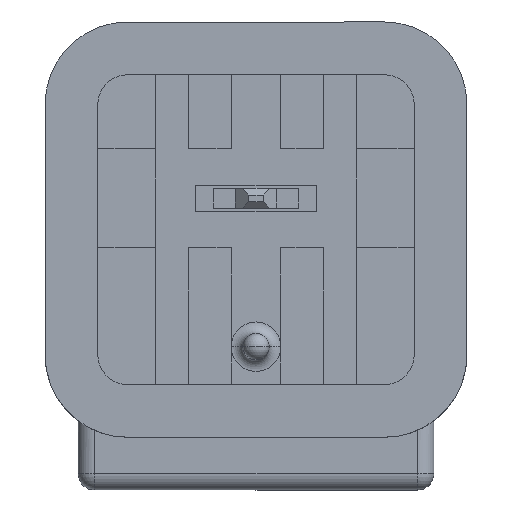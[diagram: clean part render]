
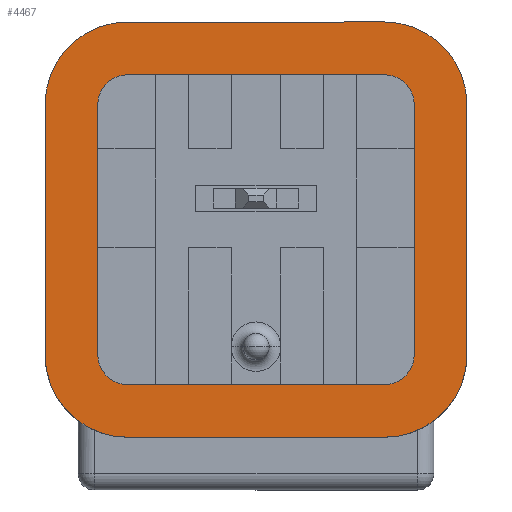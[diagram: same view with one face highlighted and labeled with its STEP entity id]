
A CAD part, front view. The second image highlights one B-rep face of the part: STEP entity #4467.
In plain terms, the highlighted planar face has unit normal (0, -1, 0).
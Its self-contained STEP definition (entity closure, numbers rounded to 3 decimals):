
#14 = LINE ( 'NONE', #4361, #474 ) ;
#16 = AXIS2_PLACEMENT_3D ( 'NONE', #4347, #647, #1285 ) ;
#30 = DIRECTION ( 'NONE',  ( 1., 0., 0. ) ) ;
#80 = EDGE_CURVE ( 'NONE', #1149, #186, #4325, .T. ) ;
#155 = DIRECTION ( 'NONE',  ( 0., -1., 0. ) ) ;
#169 = CIRCLE ( 'NONE', #16, 2.5 ) ;
#186 = VERTEX_POINT ( 'NONE', #326 ) ;
#187 = DIRECTION ( 'NONE',  ( 0., -1., 0. ) ) ;
#201 = EDGE_CURVE ( 'NONE', #4048, #1997, #14, .T. ) ;
#203 = ORIENTED_EDGE ( 'NONE', *, *, #2578, .F. ) ;
#245 = EDGE_LOOP ( 'NONE', ( #2085, #2388, #3092, #3180, #2538, #203, #2863, #3903 ) ) ;
#286 = CARTESIAN_POINT ( 'NONE',  ( -3.9, 0., -10.1 ) ) ;
#326 = CARTESIAN_POINT ( 'NONE',  ( 4.8, 0., -10.1 ) ) ;
#366 = CARTESIAN_POINT ( 'NONE',  ( 3.9, 0., -1.6 ) ) ;
#381 = CIRCLE ( 'NONE', #2443, 0.9 ) ;
#398 = VERTEX_POINT ( 'NONE', #4188 ) ;
#442 = VECTOR ( 'NONE', #2533, 1000. ) ;
#455 = EDGE_CURVE ( 'NONE', #3183, #1188, #4407, .T. ) ;
#460 = EDGE_CURVE ( 'NONE', #2556, #1149, #1193, .T. ) ;
#474 = VECTOR ( 'NONE', #3234, 1000. ) ;
#511 = VERTEX_POINT ( 'NONE', #2520 ) ;
#518 = ORIENTED_EDGE ( 'NONE', *, *, #4164, .F. ) ;
#536 = EDGE_CURVE ( 'NONE', #1997, #2963, #169, .T. ) ;
#548 = EDGE_CURVE ( 'NONE', #3319, #3502, #2851, .T. ) ;
#550 = AXIS2_PLACEMENT_3D ( 'NONE', #1909, #1558, #3824 ) ;
#595 = CARTESIAN_POINT ( 'NONE',  ( -3.9, 0., 0. ) ) ;
#647 = DIRECTION ( 'NONE',  ( 0., 1., 0. ) ) ;
#655 = EDGE_CURVE ( 'NONE', #1188, #3223, #761, .T. ) ;
#664 = CARTESIAN_POINT ( 'NONE',  ( -3.9, 0., -2.5 ) ) ;
#685 = EDGE_CURVE ( 'NONE', #2597, #398, #2942, .T. ) ;
#751 = ORIENTED_EDGE ( 'NONE', *, *, #3292, .F. ) ;
#761 = LINE ( 'NONE', #366, #1390 ) ;
#763 = CARTESIAN_POINT ( 'NONE',  ( 3.9, 0., -10.1 ) ) ;
#854 = DIRECTION ( 'NONE',  ( 1., 0., 0. ) ) ;
#877 = CARTESIAN_POINT ( 'NONE',  ( 3.9, 0., -1.6 ) ) ;
#903 = DIRECTION ( 'NONE',  ( 0., 1., 0. ) ) ;
#922 = EDGE_CURVE ( 'NONE', #3730, #4048, #2469, .T. ) ;
#946 = VERTEX_POINT ( 'NONE', #1386 ) ;
#964 = PLANE ( 'NONE',  #2120 ) ;
#981 = CARTESIAN_POINT ( 'NONE',  ( -3.9, 0., -12.6 ) ) ;
#999 = CIRCLE ( 'NONE', #2612, 2.5 ) ;
#1025 = CARTESIAN_POINT ( 'NONE',  ( -3.9, 0., -11. ) ) ;
#1032 = DIRECTION ( 'NONE',  ( -1., 0., 0. ) ) ;
#1072 = CARTESIAN_POINT ( 'NONE',  ( 6.4, 0., -10.1 ) ) ;
#1113 = VECTOR ( 'NONE', #4657, 1000. ) ;
#1137 = CARTESIAN_POINT ( 'NONE',  ( 6.4, 0., -2.5 ) ) ;
#1149 = VERTEX_POINT ( 'NONE', #1151 ) ;
#1151 = CARTESIAN_POINT ( 'NONE',  ( 3.9, 0., -11. ) ) ;
#1188 = VERTEX_POINT ( 'NONE', #877 ) ;
#1193 = LINE ( 'NONE', #4140, #3629 ) ;
#1254 = ORIENTED_EDGE ( 'NONE', *, *, #548, .F. ) ;
#1285 = DIRECTION ( 'NONE',  ( 1., 0., 0. ) ) ;
#1311 = DIRECTION ( 'NONE',  ( -1., 0., 0. ) ) ;
#1313 = CARTESIAN_POINT ( 'NONE',  ( -6.4, 0., -10.1 ) ) ;
#1386 = CARTESIAN_POINT ( 'NONE',  ( 6.4, 0., -10.1 ) ) ;
#1390 = VECTOR ( 'NONE', #2159, 1000. ) ;
#1432 = ORIENTED_EDGE ( 'NONE', *, *, #922, .F. ) ;
#1470 = CIRCLE ( 'NONE', #4695, 0.9 ) ;
#1491 = LINE ( 'NONE', #4414, #3271 ) ;
#1503 = CARTESIAN_POINT ( 'NONE',  ( -3.9, 0., 0. ) ) ;
#1558 = DIRECTION ( 'NONE',  ( 0., -1., 0. ) ) ;
#1606 = LINE ( 'NONE', #595, #1962 ) ;
#1729 = CARTESIAN_POINT ( 'NONE',  ( -3.9, 0., -1.6 ) ) ;
#1766 = DIRECTION ( 'NONE',  ( -1., 0., 0. ) ) ;
#1781 = DIRECTION ( 'NONE',  ( 1., 0., 0. ) ) ;
#1788 = ORIENTED_EDGE ( 'NONE', *, *, #2495, .F. ) ;
#1827 = CARTESIAN_POINT ( 'NONE',  ( 3.9, 0., -10.1 ) ) ;
#1868 = DIRECTION ( 'NONE',  ( 0., 0., 1. ) ) ;
#1909 = CARTESIAN_POINT ( 'NONE',  ( 3.9, 0., -2.5 ) ) ;
#1962 = VECTOR ( 'NONE', #854, 1000. ) ;
#1997 = VERTEX_POINT ( 'NONE', #4425 ) ;
#2007 = VECTOR ( 'NONE', #3643, 1000. ) ;
#2056 = CARTESIAN_POINT ( 'NONE',  ( 3.9, 0., -10.1 ) ) ;
#2084 = ORIENTED_EDGE ( 'NONE', *, *, #3995, .F. ) ;
#2085 = ORIENTED_EDGE ( 'NONE', *, *, #3928, .F. ) ;
#2120 = AXIS2_PLACEMENT_3D ( 'NONE', #1827, #2476, #1781 ) ;
#2159 = DIRECTION ( 'NONE',  ( -1., 0., 0. ) ) ;
#2295 = DIRECTION ( 'NONE',  ( 1., 0., 0. ) ) ;
#2333 = CARTESIAN_POINT ( 'NONE',  ( 4.8, 0., -2.5 ) ) ;
#2388 = ORIENTED_EDGE ( 'NONE', *, *, #80, .F. ) ;
#2443 = AXIS2_PLACEMENT_3D ( 'NONE', #3805, #155, #4618 ) ;
#2469 = CIRCLE ( 'NONE', #3868, 2.5 ) ;
#2476 = DIRECTION ( 'NONE',  ( 0., 1., 0. ) ) ;
#2495 = EDGE_CURVE ( 'NONE', #946, #511, #999, .T. ) ;
#2520 = CARTESIAN_POINT ( 'NONE',  ( 3.9, 0., -12.6 ) ) ;
#2529 = ORIENTED_EDGE ( 'NONE', *, *, #536, .F. ) ;
#2533 = DIRECTION ( 'NONE',  ( 0., 0., -1. ) ) ;
#2538 = ORIENTED_EDGE ( 'NONE', *, *, #685, .F. ) ;
#2556 = VERTEX_POINT ( 'NONE', #1025 ) ;
#2562 = CARTESIAN_POINT ( 'NONE',  ( -4.8, 0., -2.5 ) ) ;
#2578 = EDGE_CURVE ( 'NONE', #3223, #2597, #1470, .T. ) ;
#2597 = VERTEX_POINT ( 'NONE', #2562 ) ;
#2612 = AXIS2_PLACEMENT_3D ( 'NONE', #763, #903, #30 ) ;
#2658 = DIRECTION ( 'NONE',  ( 0., -1., 0. ) ) ;
#2686 = EDGE_CURVE ( 'NONE', #398, #2556, #381, .T. ) ;
#2697 = AXIS2_PLACEMENT_3D ( 'NONE', #2056, #187, #1311 ) ;
#2797 = FACE_BOUND ( 'NONE', #245, .T. ) ;
#2851 = CIRCLE ( 'NONE', #3400, 2.5 ) ;
#2863 = ORIENTED_EDGE ( 'NONE', *, *, #655, .F. ) ;
#2864 = LINE ( 'NONE', #4634, #1113 ) ;
#2942 = LINE ( 'NONE', #3672, #2007 ) ;
#2963 = VERTEX_POINT ( 'NONE', #1503 ) ;
#3092 = ORIENTED_EDGE ( 'NONE', *, *, #460, .F. ) ;
#3180 = ORIENTED_EDGE ( 'NONE', *, *, #2686, .F. ) ;
#3183 = VERTEX_POINT ( 'NONE', #2333 ) ;
#3223 = VERTEX_POINT ( 'NONE', #1729 ) ;
#3234 = DIRECTION ( 'NONE',  ( 0., 0., 1. ) ) ;
#3249 = CARTESIAN_POINT ( 'NONE',  ( 3.9, 0., 0. ) ) ;
#3271 = VECTOR ( 'NONE', #1868, 1000. ) ;
#3292 = EDGE_CURVE ( 'NONE', #511, #3730, #2864, .T. ) ;
#3319 = VERTEX_POINT ( 'NONE', #3249 ) ;
#3400 = AXIS2_PLACEMENT_3D ( 'NONE', #3846, #4569, #1032 ) ;
#3502 = VERTEX_POINT ( 'NONE', #1137 ) ;
#3612 = EDGE_LOOP ( 'NONE', ( #1788, #518, #1254, #2084, #2529, #4139, #1432, #751 ) ) ;
#3629 = VECTOR ( 'NONE', #2295, 1000. ) ;
#3643 = DIRECTION ( 'NONE',  ( 0., 0., -1. ) ) ;
#3672 = CARTESIAN_POINT ( 'NONE',  ( -4.8, 0., -2.5 ) ) ;
#3730 = VERTEX_POINT ( 'NONE', #981 ) ;
#3805 = CARTESIAN_POINT ( 'NONE',  ( -3.9, 0., -10.1 ) ) ;
#3824 = DIRECTION ( 'NONE',  ( -1., 0., 0. ) ) ;
#3846 = CARTESIAN_POINT ( 'NONE',  ( 3.9, 0., -2.5 ) ) ;
#3868 = AXIS2_PLACEMENT_3D ( 'NONE', #286, #4340, #3925 ) ;
#3903 = ORIENTED_EDGE ( 'NONE', *, *, #455, .F. ) ;
#3925 = DIRECTION ( 'NONE',  ( -1., 0., 0. ) ) ;
#3928 = EDGE_CURVE ( 'NONE', #186, #3183, #1491, .T. ) ;
#3995 = EDGE_CURVE ( 'NONE', #2963, #3319, #1606, .T. ) ;
#4048 = VERTEX_POINT ( 'NONE', #1313 ) ;
#4139 = ORIENTED_EDGE ( 'NONE', *, *, #201, .F. ) ;
#4140 = CARTESIAN_POINT ( 'NONE',  ( -3.9, 0., -11. ) ) ;
#4164 = EDGE_CURVE ( 'NONE', #3502, #946, #4386, .T. ) ;
#4188 = CARTESIAN_POINT ( 'NONE',  ( -4.8, 0., -10.1 ) ) ;
#4280 = FACE_OUTER_BOUND ( 'NONE', #3612, .T. ) ;
#4325 = CIRCLE ( 'NONE', #2697, 0.9 ) ;
#4340 = DIRECTION ( 'NONE',  ( 0., 1., 0. ) ) ;
#4347 = CARTESIAN_POINT ( 'NONE',  ( -3.9, 0., -2.5 ) ) ;
#4361 = CARTESIAN_POINT ( 'NONE',  ( -6.4, 0., -10.1 ) ) ;
#4386 = LINE ( 'NONE', #1072, #442 ) ;
#4407 = CIRCLE ( 'NONE', #550, 0.9 ) ;
#4414 = CARTESIAN_POINT ( 'NONE',  ( 4.8, 0., -10.1 ) ) ;
#4425 = CARTESIAN_POINT ( 'NONE',  ( -6.4, 0., -2.5 ) ) ;
#4467 = ADVANCED_FACE ( 'NONE', ( #2797, #4280 ), #964, .F. ) ;
#4569 = DIRECTION ( 'NONE',  ( 0., 1., 0. ) ) ;
#4618 = DIRECTION ( 'NONE',  ( -1., 0., 0. ) ) ;
#4634 = CARTESIAN_POINT ( 'NONE',  ( -3.9, 0., -12.6 ) ) ;
#4657 = DIRECTION ( 'NONE',  ( -1., 0., 0. ) ) ;
#4695 = AXIS2_PLACEMENT_3D ( 'NONE', #664, #2658, #1766 ) ;
